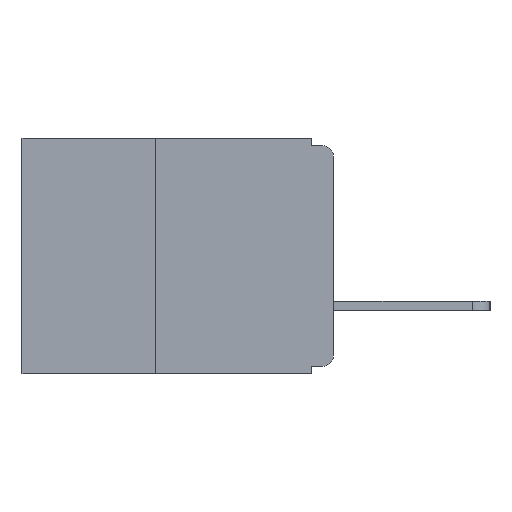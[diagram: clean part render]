
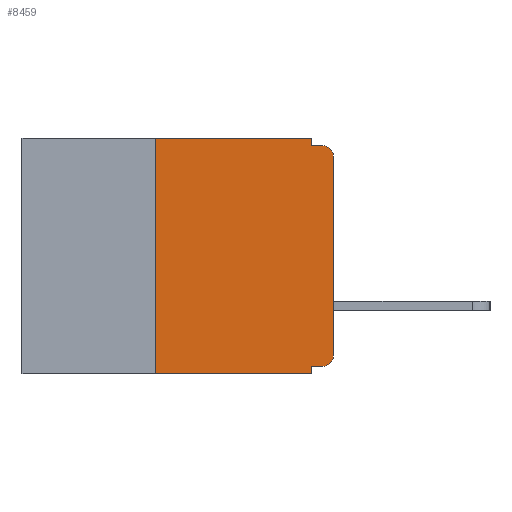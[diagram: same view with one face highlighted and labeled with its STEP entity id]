
A CAD part, left-side view. The second image highlights one B-rep face of the part: STEP entity #8459.
In plain terms, the highlighted planar face has unit normal (-1, 0, 0).
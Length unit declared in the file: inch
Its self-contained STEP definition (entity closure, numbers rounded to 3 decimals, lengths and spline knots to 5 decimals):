
#55 = LINE ( 'NONE', #14528, #2754 ) ;
#131 = DIRECTION ( 'NONE',  ( 0., 0., -1. ) ) ;
#556 = DIRECTION ( 'NONE',  ( 0., -1., 0. ) ) ;
#797 = AXIS2_PLACEMENT_3D ( 'NONE', #3420, #6153, #16861 ) ;
#1227 = ORIENTED_EDGE ( 'NONE', *, *, #2907, .F. ) ;
#1307 = DIRECTION ( 'NONE',  ( 1., 0., 0. ) ) ;
#1368 = CARTESIAN_POINT ( 'NONE',  ( 0., 0.031, 0. ) ) ;
#1411 = CARTESIAN_POINT ( 'NONE',  ( 0., 0.25, -0.33 ) ) ;
#1612 = AXIS2_PLACEMENT_3D ( 'NONE', #10668, #1307, #131 ) ;
#1912 = CARTESIAN_POINT ( 'NONE',  ( 0., 0.015, -0.01 ) ) ;
#2050 = VECTOR ( 'NONE', #5264, 39.37008 ) ;
#2078 = DIRECTION ( 'NONE',  ( 0., 0., -1. ) ) ;
#2091 = VERTEX_POINT ( 'NONE', #13683 ) ;
#2123 = CARTESIAN_POINT ( 'NONE',  ( 0., 0.031, -0.33 ) ) ;
#2443 = VECTOR ( 'NONE', #8758, 39.37008 ) ;
#2523 = VERTEX_POINT ( 'NONE', #16997 ) ;
#2577 = EDGE_CURVE ( 'NONE', #5972, #2523, #12983, .T. ) ;
#2582 = VERTEX_POINT ( 'NONE', #5613 ) ;
#2754 = VECTOR ( 'NONE', #11851, 39.37008 ) ;
#2907 = EDGE_CURVE ( 'NONE', #9779, #2582, #55, .T. ) ;
#3353 = EDGE_CURVE ( 'NONE', #15063, #7217, #4104, .T. ) ;
#3420 = CARTESIAN_POINT ( 'NONE',  ( 0., 0.015, -0.025 ) ) ;
#3437 = ORIENTED_EDGE ( 'NONE', *, *, #4421, .F. ) ;
#3454 = ORIENTED_EDGE ( 'NONE', *, *, #2577, .F. ) ;
#3968 = EDGE_CURVE ( 'NONE', #15063, #5547, #16990, .T. ) ;
#4104 = LINE ( 'NONE', #1411, #16953 ) ;
#4177 = CARTESIAN_POINT ( 'NONE',  ( 0., 0.437, 0. ) ) ;
#4421 = EDGE_CURVE ( 'NONE', #2582, #5547, #14262, .T. ) ;
#4436 = CARTESIAN_POINT ( 'NONE',  ( 0., 0., 0. ) ) ;
#5132 = EDGE_CURVE ( 'NONE', #2091, #14606, #9459, .T. ) ;
#5264 = DIRECTION ( 'NONE',  ( 0., -1., 0. ) ) ;
#5373 = ORIENTED_EDGE ( 'NONE', *, *, #10375, .F. ) ;
#5547 = VERTEX_POINT ( 'NONE', #2123 ) ;
#5613 = CARTESIAN_POINT ( 'NONE',  ( 0., 0.031, -0.32 ) ) ;
#5972 = VERTEX_POINT ( 'NONE', #10634 ) ;
#6097 = VECTOR ( 'NONE', #12401, 39.37008 ) ;
#6153 = DIRECTION ( 'NONE',  ( -1., 0., 0. ) ) ;
#6420 = LINE ( 'NONE', #13314, #2050 ) ;
#7217 = VERTEX_POINT ( 'NONE', #11530 ) ;
#7569 = DIRECTION ( 'NONE',  ( -1., 0., 0. ) ) ;
#8459 = ADVANCED_FACE ( 'NONE', ( #15125 ), #13172, .F. ) ;
#8758 = DIRECTION ( 'NONE',  ( 0., -1., 0. ) ) ;
#9081 = LINE ( 'NONE', #4177, #2443 ) ;
#9186 = ORIENTED_EDGE ( 'NONE', *, *, #5132, .T. ) ;
#9327 = EDGE_LOOP ( 'NONE', ( #16171, #9186, #16198, #3454, #5373, #16407, #12162, #3437, #1227, #16203 ) ) ;
#9428 = DIRECTION ( 'NONE',  ( 0., 0., 1. ) ) ;
#9459 = CIRCLE ( 'NONE', #797, 0.015 ) ;
#9538 = CARTESIAN_POINT ( 'NONE',  ( 0., 0.25, -0.33 ) ) ;
#9563 = DIRECTION ( 'NONE',  ( 0., 0., -1. ) ) ;
#9779 = VERTEX_POINT ( 'NONE', #10902 ) ;
#10058 = LINE ( 'NONE', #4436, #6097 ) ;
#10375 = EDGE_CURVE ( 'NONE', #7217, #5972, #9081, .T. ) ;
#10634 = CARTESIAN_POINT ( 'NONE',  ( 0., 0.031, 0. ) ) ;
#10668 = CARTESIAN_POINT ( 'NONE',  ( 0., 0.437, 0. ) ) ;
#10902 = CARTESIAN_POINT ( 'NONE',  ( 0., 0.015, -0.32 ) ) ;
#11332 = CARTESIAN_POINT ( 'NONE',  ( 0., 0., -0.305 ) ) ;
#11388 = CARTESIAN_POINT ( 'NONE',  ( 0., 0.437, -0.33 ) ) ;
#11530 = CARTESIAN_POINT ( 'NONE',  ( 0., 0.25, 0. ) ) ;
#11851 = DIRECTION ( 'NONE',  ( 0., 1., 0. ) ) ;
#12162 = ORIENTED_EDGE ( 'NONE', *, *, #3968, .T. ) ;
#12401 = DIRECTION ( 'NONE',  ( 0., 0., 1. ) ) ;
#12857 = EDGE_CURVE ( 'NONE', #16148, #2091, #10058, .T. ) ;
#12983 = LINE ( 'NONE', #1368, #14395 ) ;
#13172 = PLANE ( 'NONE',  #1612 ) ;
#13314 = CARTESIAN_POINT ( 'NONE',  ( 0., 0., -0.01 ) ) ;
#13683 = CARTESIAN_POINT ( 'NONE',  ( 0., 0., -0.025 ) ) ;
#13691 = VECTOR ( 'NONE', #556, 39.37008 ) ;
#14120 = CARTESIAN_POINT ( 'NONE',  ( 0., 0.031, -0.33 ) ) ;
#14262 = LINE ( 'NONE', #14120, #14673 ) ;
#14395 = VECTOR ( 'NONE', #9563, 39.37008 ) ;
#14528 = CARTESIAN_POINT ( 'NONE',  ( 0., 0., -0.32 ) ) ;
#14606 = VERTEX_POINT ( 'NONE', #1912 ) ;
#14673 = VECTOR ( 'NONE', #2078, 39.37008 ) ;
#15063 = VERTEX_POINT ( 'NONE', #9538 ) ;
#15125 = FACE_OUTER_BOUND ( 'NONE', #9327, .T. ) ;
#15409 = AXIS2_PLACEMENT_3D ( 'NONE', #15469, #7569, #16884 ) ;
#15469 = CARTESIAN_POINT ( 'NONE',  ( 0., 0.015, -0.305 ) ) ;
#15509 = EDGE_CURVE ( 'NONE', #2523, #14606, #6420, .T. ) ;
#16148 = VERTEX_POINT ( 'NONE', #11332 ) ;
#16171 = ORIENTED_EDGE ( 'NONE', *, *, #12857, .T. ) ;
#16198 = ORIENTED_EDGE ( 'NONE', *, *, #15509, .F. ) ;
#16203 = ORIENTED_EDGE ( 'NONE', *, *, #17070, .T. ) ;
#16407 = ORIENTED_EDGE ( 'NONE', *, *, #3353, .F. ) ;
#16861 = DIRECTION ( 'NONE',  ( 0., 0., -1. ) ) ;
#16884 = DIRECTION ( 'NONE',  ( 0., 0., -1. ) ) ;
#16953 = VECTOR ( 'NONE', #9428, 39.37008 ) ;
#16990 = LINE ( 'NONE', #11388, #13691 ) ;
#16997 = CARTESIAN_POINT ( 'NONE',  ( 0., 0.031, -0.01 ) ) ;
#17070 = EDGE_CURVE ( 'NONE', #9779, #16148, #17243, .T. ) ;
#17243 = CIRCLE ( 'NONE', #15409, 0.015 ) ;
